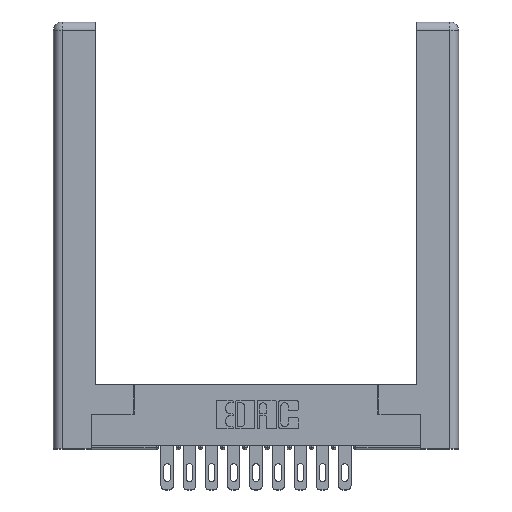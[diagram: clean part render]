
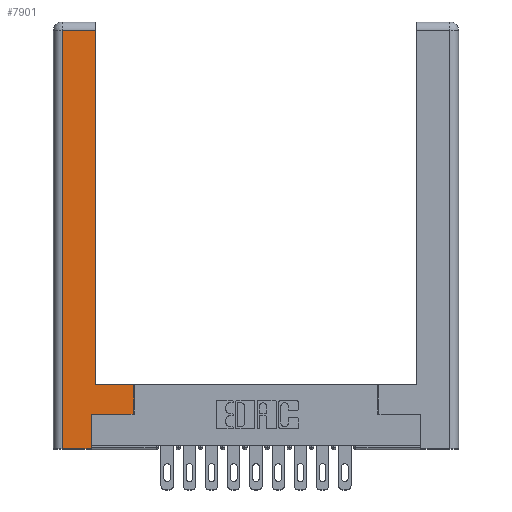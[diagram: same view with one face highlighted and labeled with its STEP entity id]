
A CAD part, top view. The second image highlights one B-rep face of the part: STEP entity #7901.
In plain terms, the highlighted planar face has unit normal (0, 0, 1).
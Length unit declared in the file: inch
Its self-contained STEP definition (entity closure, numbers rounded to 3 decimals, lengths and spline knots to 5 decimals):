
#217 = EDGE_CURVE ( 'NONE', #3494, #2499, #6670, .T. ) ;
#589 = DIRECTION ( 'NONE',  ( -1., 0., 0. ) ) ;
#1312 = VECTOR ( 'NONE', #9439, 39.37008 ) ;
#1478 = ORIENTED_EDGE ( 'NONE', *, *, #2521, .T. ) ;
#1488 = CARTESIAN_POINT ( 'NONE',  ( 0.295, 3., 0. ) ) ;
#1701 = CARTESIAN_POINT ( 'NONE',  ( 0.295, 0.45, 0. ) ) ;
#1777 = LINE ( 'NONE', #1488, #11265 ) ;
#1788 = PLANE ( 'NONE',  #14913 ) ;
#1889 = VERTEX_POINT ( 'NONE', #4020 ) ;
#1897 = DIRECTION ( 'NONE',  ( 1., 0., 0. ) ) ;
#1967 = EDGE_CURVE ( 'NONE', #1889, #14043, #13965, .T. ) ;
#2021 = ORIENTED_EDGE ( 'NONE', *, *, #10214, .T. ) ;
#2232 = LINE ( 'NONE', #6396, #8167 ) ;
#2499 = VERTEX_POINT ( 'NONE', #6229 ) ;
#2521 = EDGE_CURVE ( 'NONE', #14043, #13037, #9972, .T. ) ;
#2714 = ORIENTED_EDGE ( 'NONE', *, *, #217, .T. ) ;
#3134 = CARTESIAN_POINT ( 'NONE',  ( 0.565, 0.245, 0. ) ) ;
#3357 = DIRECTION ( 'NONE',  ( 1., 0., 0. ) ) ;
#3447 = CARTESIAN_POINT ( 'NONE',  ( 0.265, 0., 0. ) ) ;
#3494 = VERTEX_POINT ( 'NONE', #9305 ) ;
#3537 = VECTOR ( 'NONE', #12872, 39.37008 ) ;
#3994 = DIRECTION ( 'NONE',  ( 0., 1., 0. ) ) ;
#4020 = CARTESIAN_POINT ( 'NONE',  ( 0.0615, 0., 0. ) ) ;
#5408 = LINE ( 'NONE', #3134, #11277 ) ;
#5866 = ORIENTED_EDGE ( 'NONE', *, *, #1967, .T. ) ;
#6202 = ORIENTED_EDGE ( 'NONE', *, *, #7949, .T. ) ;
#6229 = CARTESIAN_POINT ( 'NONE',  ( 0.565, 0.45, 0. ) ) ;
#6396 = CARTESIAN_POINT ( 'NONE',  ( 0.0615, 0., 0. ) ) ;
#6407 = EDGE_CURVE ( 'NONE', #2499, #8536, #8361, .T. ) ;
#6615 = CARTESIAN_POINT ( 'NONE',  ( 0., 0., 0. ) ) ;
#6647 = EDGE_CURVE ( 'NONE', #6783, #1889, #2232, .T. ) ;
#6670 = LINE ( 'NONE', #12961, #3537 ) ;
#6783 = VERTEX_POINT ( 'NONE', #10216 ) ;
#6808 = VECTOR ( 'NONE', #8896, 39.37008 ) ;
#6878 = VERTEX_POINT ( 'NONE', #10372 ) ;
#7781 = DIRECTION ( 'NONE',  ( 0., 0., -1. ) ) ;
#7901 = ADVANCED_FACE ( 'NONE', ( #9272 ), #1788, .F. ) ;
#7949 = EDGE_CURVE ( 'NONE', #13037, #3494, #5408, .T. ) ;
#8167 = VECTOR ( 'NONE', #8757, 39.37008 ) ;
#8214 = CARTESIAN_POINT ( 'NONE',  ( 0.0615, 2.94, 0. ) ) ;
#8361 = LINE ( 'NONE', #12022, #14263 ) ;
#8403 = EDGE_CURVE ( 'NONE', #8536, #6878, #1777, .T. ) ;
#8536 = VERTEX_POINT ( 'NONE', #1701 ) ;
#8757 = DIRECTION ( 'NONE',  ( 0., -1., 0. ) ) ;
#8896 = DIRECTION ( 'NONE',  ( 0., 1., 0. ) ) ;
#9272 = FACE_OUTER_BOUND ( 'NONE', #9316, .T. ) ;
#9305 = CARTESIAN_POINT ( 'NONE',  ( 0.565, 0.245, 0. ) ) ;
#9316 = EDGE_LOOP ( 'NONE', ( #10790, #2021, #14054, #5866, #1478, #6202, #2714, #10158 ) ) ;
#9439 = DIRECTION ( 'NONE',  ( -1., 0., 0. ) ) ;
#9972 = LINE ( 'NONE', #11954, #6808 ) ;
#10158 = ORIENTED_EDGE ( 'NONE', *, *, #6407, .T. ) ;
#10214 = EDGE_CURVE ( 'NONE', #6878, #6783, #10845, .T. ) ;
#10216 = CARTESIAN_POINT ( 'NONE',  ( 0.0615, 2.94, 0. ) ) ;
#10372 = CARTESIAN_POINT ( 'NONE',  ( 0.295, 2.94, 0. ) ) ;
#10790 = ORIENTED_EDGE ( 'NONE', *, *, #8403, .T. ) ;
#10845 = LINE ( 'NONE', #8214, #1312 ) ;
#10866 = VECTOR ( 'NONE', #3357, 39.37008 ) ;
#11052 = CARTESIAN_POINT ( 'NONE',  ( 0.265, 0., 0. ) ) ;
#11265 = VECTOR ( 'NONE', #3994, 39.37008 ) ;
#11277 = VECTOR ( 'NONE', #1897, 39.37008 ) ;
#11954 = CARTESIAN_POINT ( 'NONE',  ( 0.265, 0.245, 0. ) ) ;
#12022 = CARTESIAN_POINT ( 'NONE',  ( 0.295, 0.45, 0. ) ) ;
#12872 = DIRECTION ( 'NONE',  ( 0., 1., 0. ) ) ;
#12961 = CARTESIAN_POINT ( 'NONE',  ( 0.565, 0.45, 0. ) ) ;
#13037 = VERTEX_POINT ( 'NONE', #14987 ) ;
#13191 = DIRECTION ( 'NONE',  ( -1., 0., 0. ) ) ;
#13965 = LINE ( 'NONE', #3447, #10866 ) ;
#14043 = VERTEX_POINT ( 'NONE', #11052 ) ;
#14054 = ORIENTED_EDGE ( 'NONE', *, *, #6647, .T. ) ;
#14263 = VECTOR ( 'NONE', #13191, 39.37008 ) ;
#14913 = AXIS2_PLACEMENT_3D ( 'NONE', #6615, #7781, #589 ) ;
#14987 = CARTESIAN_POINT ( 'NONE',  ( 0.265, 0.245, 0. ) ) ;
